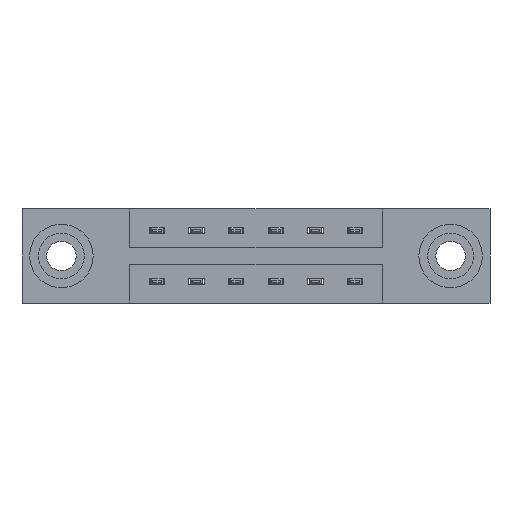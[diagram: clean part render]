
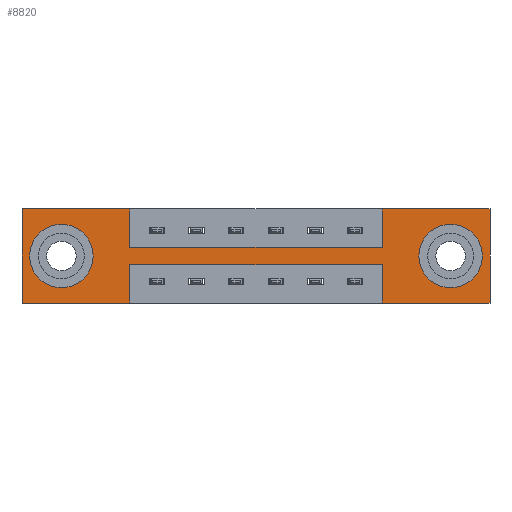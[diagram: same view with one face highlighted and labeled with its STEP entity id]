
A CAD part, front view. The second image highlights one B-rep face of the part: STEP entity #8820.
In plain terms, the highlighted planar face has unit normal (0, -1, 0).
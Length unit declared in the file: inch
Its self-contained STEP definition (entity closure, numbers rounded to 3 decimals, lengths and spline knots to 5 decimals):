
#49 = CIRCLE ( 'NONE', #8542, 0.078 ) ;
#128 = ORIENTED_EDGE ( 'NONE', *, *, #9217, .T. ) ;
#180 = VECTOR ( 'NONE', #9257, 39.37008 ) ;
#189 = CARTESIAN_POINT ( 'NONE',  ( 0.425, 0., -0.22 ) ) ;
#258 = CIRCLE ( 'NONE', #8347, 0.078 ) ;
#320 = LINE ( 'NONE', #8141, #8284 ) ;
#349 = ORIENTED_EDGE ( 'NONE', *, *, #5561, .F. ) ;
#410 = CARTESIAN_POINT ( 'NONE',  ( 0.425, 0., 0. ) ) ;
#430 = VECTOR ( 'NONE', #556, 39.37008 ) ;
#556 = DIRECTION ( 'NONE',  ( -1., 0., 0. ) ) ;
#642 = CARTESIAN_POINT ( 'NONE',  ( 0., 0., 0. ) ) ;
#652 = EDGE_CURVE ( 'NONE', #1084, #941, #5276, .T. ) ;
#705 = CARTESIAN_POINT ( 'NONE',  ( 1.417, 0., -0.15 ) ) ;
#794 = DIRECTION ( 'NONE',  ( 1., 0., 0. ) ) ;
#941 = VERTEX_POINT ( 'NONE', #6321 ) ;
#974 = DIRECTION ( 'NONE',  ( 0., 0., 1. ) ) ;
#1042 = EDGE_LOOP ( 'NONE', ( #7642, #7510, #349, #8139, #8305, #8385, #4494, #9471, #9432, #8017, #1280, #7018 ) ) ;
#1051 = CARTESIAN_POINT ( 'NONE',  ( 0., 0., 0. ) ) ;
#1061 = DIRECTION ( 'NONE',  ( 1., 0., 0. ) ) ;
#1084 = VERTEX_POINT ( 'NONE', #6398 ) ;
#1259 = VERTEX_POINT ( 'NONE', #8174 ) ;
#1280 = ORIENTED_EDGE ( 'NONE', *, *, #5368, .F. ) ;
#1479 = CARTESIAN_POINT ( 'NONE',  ( 1.417, 0., -0.37 ) ) ;
#1523 = LINE ( 'NONE', #642, #3435 ) ;
#1709 = CARTESIAN_POINT ( 'NONE',  ( 0.155, 0., -0.185 ) ) ;
#1742 = VERTEX_POINT ( 'NONE', #2032 ) ;
#1747 = CARTESIAN_POINT ( 'NONE',  ( 0., 0., -0.37 ) ) ;
#1780 = CARTESIAN_POINT ( 'NONE',  ( 1.687, 0., -0.185 ) ) ;
#1803 = VECTOR ( 'NONE', #8924, 39.37008 ) ;
#1935 = LINE ( 'NONE', #3160, #6013 ) ;
#1939 = VERTEX_POINT ( 'NONE', #410 ) ;
#1978 = DIRECTION ( 'NONE',  ( 0., 0., -1. ) ) ;
#2022 = VERTEX_POINT ( 'NONE', #1479 ) ;
#2032 = CARTESIAN_POINT ( 'NONE',  ( 1.842, 0., 0. ) ) ;
#2059 = PLANE ( 'NONE',  #8800 ) ;
#2081 = EDGE_CURVE ( 'NONE', #941, #1084, #49, .T. ) ;
#2127 = CARTESIAN_POINT ( 'NONE',  ( 0., 0., -0.37 ) ) ;
#2230 = DIRECTION ( 'NONE',  ( 0., 0., -1. ) ) ;
#2251 = DIRECTION ( 'NONE',  ( 0., 1., 0. ) ) ;
#2289 = DIRECTION ( 'NONE',  ( 0., 0., 1. ) ) ;
#2332 = DIRECTION ( 'NONE',  ( 0., 1., 0. ) ) ;
#2336 = DIRECTION ( 'NONE',  ( 0., 0., -1. ) ) ;
#2362 = LINE ( 'NONE', #2578, #9766 ) ;
#2376 = VERTEX_POINT ( 'NONE', #2979 ) ;
#2410 = DIRECTION ( 'NONE',  ( 0., -1., 0. ) ) ;
#2437 = DIRECTION ( 'NONE',  ( 0., 1., 0. ) ) ;
#2463 = VERTEX_POINT ( 'NONE', #4032 ) ;
#2578 = CARTESIAN_POINT ( 'NONE',  ( 1.842, 0., 0. ) ) ;
#2672 = FACE_BOUND ( 'NONE', #4106, .T. ) ;
#2700 = EDGE_CURVE ( 'NONE', #2985, #1742, #9450, .T. ) ;
#2741 = DIRECTION ( 'NONE',  ( -1., 0., 0. ) ) ;
#2840 = VERTEX_POINT ( 'NONE', #705 ) ;
#2849 = LINE ( 'NONE', #1747, #430 ) ;
#2870 = DIRECTION ( 'NONE',  ( 0., 1., 0. ) ) ;
#2979 = CARTESIAN_POINT ( 'NONE',  ( 0.425, 0., -0.15 ) ) ;
#2985 = VERTEX_POINT ( 'NONE', #5447 ) ;
#3052 = VECTOR ( 'NONE', #8524, 39.37008 ) ;
#3067 = CIRCLE ( 'NONE', #8294, 0.078 ) ;
#3152 = CARTESIAN_POINT ( 'NONE',  ( 1.687, 0., -0.185 ) ) ;
#3160 = CARTESIAN_POINT ( 'NONE',  ( 0., 0., -0.37 ) ) ;
#3435 = VECTOR ( 'NONE', #794, 39.37008 ) ;
#3482 = AXIS2_PLACEMENT_3D ( 'NONE', #1780, #2437, #2336 ) ;
#3518 = CARTESIAN_POINT ( 'NONE',  ( 1.417, 0., -0.22 ) ) ;
#3693 = LINE ( 'NONE', #6566, #1803 ) ;
#3830 = EDGE_LOOP ( 'NONE', ( #6054, #128 ) ) ;
#3880 = VERTEX_POINT ( 'NONE', #3518 ) ;
#3978 = VECTOR ( 'NONE', #4027, 39.37008 ) ;
#4003 = VERTEX_POINT ( 'NONE', #4100 ) ;
#4027 = DIRECTION ( 'NONE',  ( 0., 0., 1. ) ) ;
#4032 = CARTESIAN_POINT ( 'NONE',  ( 0.155, 0., -0.263 ) ) ;
#4056 = EDGE_CURVE ( 'NONE', #2840, #2985, #9781, .T. ) ;
#4100 = CARTESIAN_POINT ( 'NONE',  ( 0.155, 0., -0.107 ) ) ;
#4106 = EDGE_LOOP ( 'NONE', ( #6448, #6406 ) ) ;
#4190 = VECTOR ( 'NONE', #974, 39.37008 ) ;
#4367 = VERTEX_POINT ( 'NONE', #7410 ) ;
#4418 = LINE ( 'NONE', #6661, #4190 ) ;
#4467 = FACE_OUTER_BOUND ( 'NONE', #1042, .T. ) ;
#4494 = ORIENTED_EDGE ( 'NONE', *, *, #4056, .F. ) ;
#4881 = EDGE_CURVE ( 'NONE', #1742, #5184, #2362, .T. ) ;
#5077 = CARTESIAN_POINT ( 'NONE',  ( 0.425, 0., -0.22 ) ) ;
#5184 = VERTEX_POINT ( 'NONE', #5356 ) ;
#5276 = CIRCLE ( 'NONE', #3482, 0.078 ) ;
#5300 = LINE ( 'NONE', #8557, #3052 ) ;
#5356 = CARTESIAN_POINT ( 'NONE',  ( 1.842, 0., -0.37 ) ) ;
#5368 = EDGE_CURVE ( 'NONE', #4367, #5554, #4418, .T. ) ;
#5447 = CARTESIAN_POINT ( 'NONE',  ( 1.417, 0., 0. ) ) ;
#5554 = VERTEX_POINT ( 'NONE', #7526 ) ;
#5561 = EDGE_CURVE ( 'NONE', #2022, #3880, #320, .T. ) ;
#5851 = CARTESIAN_POINT ( 'NONE',  ( 0.425, 0., -0.37 ) ) ;
#5862 = EDGE_CURVE ( 'NONE', #8283, #1259, #5930, .T. ) ;
#5930 = LINE ( 'NONE', #5851, #180 ) ;
#6013 = VECTOR ( 'NONE', #2741, 39.37008 ) ;
#6054 = ORIENTED_EDGE ( 'NONE', *, *, #8837, .T. ) ;
#6215 = DIRECTION ( 'NONE',  ( 0., 0., -1. ) ) ;
#6321 = CARTESIAN_POINT ( 'NONE',  ( 1.687, 0., -0.107 ) ) ;
#6398 = CARTESIAN_POINT ( 'NONE',  ( 1.687, 0., -0.263 ) ) ;
#6406 = ORIENTED_EDGE ( 'NONE', *, *, #652, .T. ) ;
#6448 = ORIENTED_EDGE ( 'NONE', *, *, #2081, .T. ) ;
#6566 = CARTESIAN_POINT ( 'NONE',  ( 0.425, 0., 0. ) ) ;
#6661 = CARTESIAN_POINT ( 'NONE',  ( 0., 0., 0. ) ) ;
#6665 = EDGE_CURVE ( 'NONE', #1259, #4367, #2849, .T. ) ;
#7018 = ORIENTED_EDGE ( 'NONE', *, *, #6665, .F. ) ;
#7132 = EDGE_CURVE ( 'NONE', #3880, #8283, #9232, .T. ) ;
#7325 = EDGE_CURVE ( 'NONE', #1939, #2376, #3693, .T. ) ;
#7402 = VECTOR ( 'NONE', #1061, 39.37008 ) ;
#7410 = CARTESIAN_POINT ( 'NONE',  ( 0., 0., -0.37 ) ) ;
#7451 = CARTESIAN_POINT ( 'NONE',  ( 0.155, 0., -0.185 ) ) ;
#7455 = DIRECTION ( 'NONE',  ( -1., 0., 0. ) ) ;
#7510 = ORIENTED_EDGE ( 'NONE', *, *, #7132, .F. ) ;
#7526 = CARTESIAN_POINT ( 'NONE',  ( 0., 0., 0. ) ) ;
#7528 = EDGE_CURVE ( 'NONE', #5184, #2022, #1935, .T. ) ;
#7642 = ORIENTED_EDGE ( 'NONE', *, *, #5862, .F. ) ;
#8017 = ORIENTED_EDGE ( 'NONE', *, *, #8690, .F. ) ;
#8073 = CARTESIAN_POINT ( 'NONE',  ( 1.417, 0., 0. ) ) ;
#8139 = ORIENTED_EDGE ( 'NONE', *, *, #7528, .F. ) ;
#8140 = DIRECTION ( 'NONE',  ( 0., 0., 1. ) ) ;
#8141 = CARTESIAN_POINT ( 'NONE',  ( 1.417, 0., -0.37 ) ) ;
#8174 = CARTESIAN_POINT ( 'NONE',  ( 0.425, 0., -0.37 ) ) ;
#8219 = FACE_BOUND ( 'NONE', #3830, .T. ) ;
#8283 = VERTEX_POINT ( 'NONE', #189 ) ;
#8284 = VECTOR ( 'NONE', #9734, 39.37008 ) ;
#8294 = AXIS2_PLACEMENT_3D ( 'NONE', #7451, #2870, #8140 ) ;
#8305 = ORIENTED_EDGE ( 'NONE', *, *, #4881, .F. ) ;
#8347 = AXIS2_PLACEMENT_3D ( 'NONE', #1709, #2332, #2289 ) ;
#8385 = ORIENTED_EDGE ( 'NONE', *, *, #2700, .F. ) ;
#8524 = DIRECTION ( 'NONE',  ( 1., 0., 0. ) ) ;
#8542 = AXIS2_PLACEMENT_3D ( 'NONE', #3152, #2251, #2230 ) ;
#8557 = CARTESIAN_POINT ( 'NONE',  ( 0.425, 0., -0.15 ) ) ;
#8690 = EDGE_CURVE ( 'NONE', #5554, #1939, #1523, .T. ) ;
#8800 = AXIS2_PLACEMENT_3D ( 'NONE', #2127, #2410, #1978 ) ;
#8820 = ADVANCED_FACE ( 'NONE', ( #2672, #8219, #4467 ), #2059, .T. ) ;
#8837 = EDGE_CURVE ( 'NONE', #4003, #2463, #258, .T. ) ;
#8924 = DIRECTION ( 'NONE',  ( 0., 0., -1. ) ) ;
#9012 = VECTOR ( 'NONE', #7455, 39.37008 ) ;
#9217 = EDGE_CURVE ( 'NONE', #2463, #4003, #3067, .T. ) ;
#9232 = LINE ( 'NONE', #5077, #9012 ) ;
#9257 = DIRECTION ( 'NONE',  ( 0., 0., -1. ) ) ;
#9432 = ORIENTED_EDGE ( 'NONE', *, *, #7325, .F. ) ;
#9450 = LINE ( 'NONE', #1051, #7402 ) ;
#9471 = ORIENTED_EDGE ( 'NONE', *, *, #9631, .F. ) ;
#9631 = EDGE_CURVE ( 'NONE', #2376, #2840, #5300, .T. ) ;
#9734 = DIRECTION ( 'NONE',  ( 0., 0., 1. ) ) ;
#9766 = VECTOR ( 'NONE', #6215, 39.37008 ) ;
#9781 = LINE ( 'NONE', #8073, #3978 ) ;
